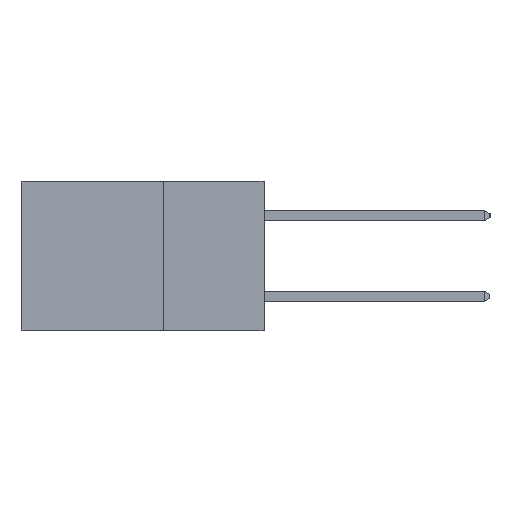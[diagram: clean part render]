
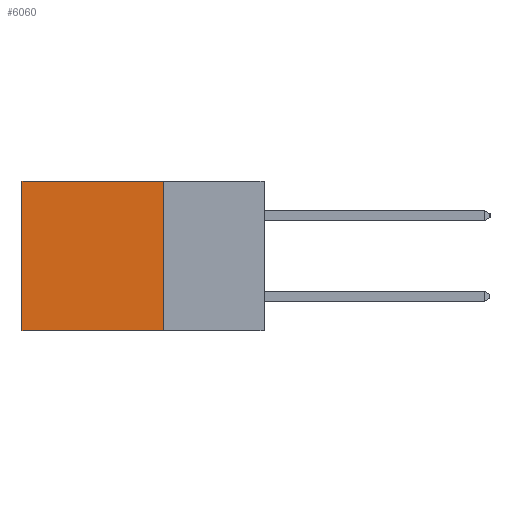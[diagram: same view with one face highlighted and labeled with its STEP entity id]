
A CAD part, left-side view. The second image highlights one B-rep face of the part: STEP entity #6060.
In plain terms, the highlighted planar face has unit normal (-1, 0, 0).
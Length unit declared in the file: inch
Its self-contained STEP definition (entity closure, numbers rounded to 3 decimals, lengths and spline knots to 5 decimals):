
#308 = ORIENTED_EDGE ( 'NONE', *, *, #14235, .F. ) ;
#443 = EDGE_LOOP ( 'NONE', ( #3474, #308, #5052, #16181 ) ) ;
#905 = CARTESIAN_POINT ( 'NONE',  ( 0.2615, 0.25, -0.37 ) ) ;
#2293 = CARTESIAN_POINT ( 'NONE',  ( 0.2615, 0.6, -0.37 ) ) ;
#3217 = CARTESIAN_POINT ( 'NONE',  ( 0.2615, 0.6, -0.37 ) ) ;
#3474 = ORIENTED_EDGE ( 'NONE', *, *, #10517, .T. ) ;
#4192 = VECTOR ( 'NONE', #10987, 39.37008 ) ;
#5052 = ORIENTED_EDGE ( 'NONE', *, *, #8163, .F. ) ;
#6060 = ADVANCED_FACE ( 'NONE', ( #11733 ), #8711, .F. ) ;
#7683 = CARTESIAN_POINT ( 'NONE',  ( 0.2615, 0.25, 0. ) ) ;
#8163 = EDGE_CURVE ( 'NONE', #20678, #21065, #18423, .T. ) ;
#8711 = PLANE ( 'NONE',  #16583 ) ;
#8776 = LINE ( 'NONE', #7683, #21677 ) ;
#9110 = CARTESIAN_POINT ( 'NONE',  ( 0.2615, 0.25, -0.37 ) ) ;
#9534 = DIRECTION ( 'NONE',  ( 0., 1., 0. ) ) ;
#10517 = EDGE_CURVE ( 'NONE', #20211, #22899, #20606, .T. ) ;
#10570 = DIRECTION ( 'NONE',  ( 0., 0., -1. ) ) ;
#10987 = DIRECTION ( 'NONE',  ( 0., 0., -1. ) ) ;
#11273 = LINE ( 'NONE', #24040, #16156 ) ;
#11478 = VECTOR ( 'NONE', #22676, 39.37008 ) ;
#11733 = FACE_OUTER_BOUND ( 'NONE', #443, .T. ) ;
#12296 = EDGE_CURVE ( 'NONE', #20678, #20211, #8776, .T. ) ;
#13120 = DIRECTION ( 'NONE',  ( 0., 1., 0. ) ) ;
#14235 = EDGE_CURVE ( 'NONE', #21065, #22899, #11273, .T. ) ;
#16156 = VECTOR ( 'NONE', #13120, 39.37008 ) ;
#16181 = ORIENTED_EDGE ( 'NONE', *, *, #12296, .T. ) ;
#16583 = AXIS2_PLACEMENT_3D ( 'NONE', #905, #21542, #10570 ) ;
#17479 = CARTESIAN_POINT ( 'NONE',  ( 0.2615, 0.25, 0. ) ) ;
#18423 = LINE ( 'NONE', #9110, #4192 ) ;
#18425 = CARTESIAN_POINT ( 'NONE',  ( 0.2615, 0.25, -0.37 ) ) ;
#20211 = VERTEX_POINT ( 'NONE', #23654 ) ;
#20606 = LINE ( 'NONE', #2293, #11478 ) ;
#20678 = VERTEX_POINT ( 'NONE', #17479 ) ;
#21065 = VERTEX_POINT ( 'NONE', #18425 ) ;
#21542 = DIRECTION ( 'NONE',  ( 1., 0., 0. ) ) ;
#21677 = VECTOR ( 'NONE', #9534, 39.37008 ) ;
#22676 = DIRECTION ( 'NONE',  ( 0., 0., -1. ) ) ;
#22899 = VERTEX_POINT ( 'NONE', #3217 ) ;
#23654 = CARTESIAN_POINT ( 'NONE',  ( 0.2615, 0.6, 0. ) ) ;
#24040 = CARTESIAN_POINT ( 'NONE',  ( 0.2615, 0.25, -0.37 ) ) ;
